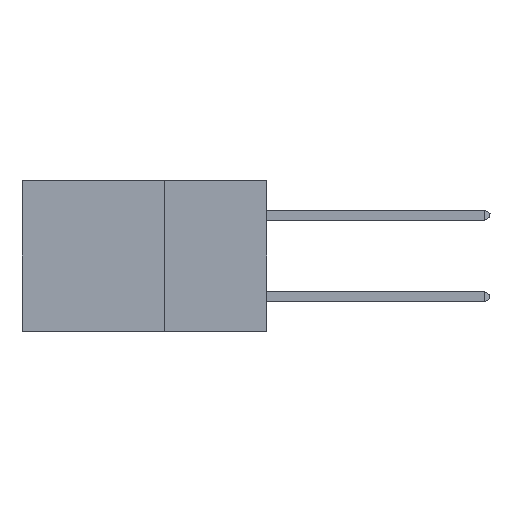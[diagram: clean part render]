
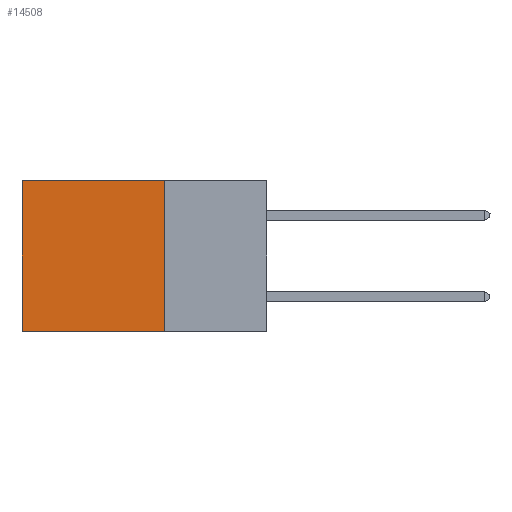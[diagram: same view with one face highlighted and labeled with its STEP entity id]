
A CAD part, left-side view. The second image highlights one B-rep face of the part: STEP entity #14508.
In plain terms, the highlighted planar face has unit normal (-1, 0, 0).
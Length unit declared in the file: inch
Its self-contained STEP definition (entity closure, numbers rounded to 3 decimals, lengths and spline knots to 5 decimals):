
#891 = LINE ( 'NONE', #15356, #12651 ) ;
#1156 = DIRECTION ( 'NONE',  ( 0., 1., 0. ) ) ;
#2074 = DIRECTION ( 'NONE',  ( 0., 1., 0. ) ) ;
#2158 = CARTESIAN_POINT ( 'NONE',  ( 0.2875, 0.25, 0. ) ) ;
#3663 = VECTOR ( 'NONE', #12455, 39.37008 ) ;
#4318 = CARTESIAN_POINT ( 'NONE',  ( 0.2875, 0.25, -0.37 ) ) ;
#5092 = LINE ( 'NONE', #8148, #12382 ) ;
#5104 = ORIENTED_EDGE ( 'NONE', *, *, #21086, .T. ) ;
#5555 = AXIS2_PLACEMENT_3D ( 'NONE', #7873, #11827, #15856 ) ;
#5577 = LINE ( 'NONE', #2158, #3663 ) ;
#7801 = VERTEX_POINT ( 'NONE', #24336 ) ;
#7873 = CARTESIAN_POINT ( 'NONE',  ( 0.2875, 0.25, 0. ) ) ;
#8148 = CARTESIAN_POINT ( 'NONE',  ( 0.2875, 0.25, 0. ) ) ;
#8924 = CARTESIAN_POINT ( 'NONE',  ( 0.2875, 0.25, -0.37 ) ) ;
#9270 = DIRECTION ( 'NONE',  ( 0., 0., -1. ) ) ;
#10845 = EDGE_CURVE ( 'NONE', #7801, #23779, #5092, .T. ) ;
#11282 = ORIENTED_EDGE ( 'NONE', *, *, #18665, .F. ) ;
#11827 = DIRECTION ( 'NONE',  ( 1., 0., 0. ) ) ;
#11918 = PLANE ( 'NONE',  #5555 ) ;
#12382 = VECTOR ( 'NONE', #2074, 39.37008 ) ;
#12455 = DIRECTION ( 'NONE',  ( 0., 0., -1. ) ) ;
#12651 = VECTOR ( 'NONE', #9270, 39.37008 ) ;
#12798 = FACE_OUTER_BOUND ( 'NONE', #18813, .T. ) ;
#14508 = ADVANCED_FACE ( 'NONE', ( #12798 ), #11918, .F. ) ;
#14721 = CARTESIAN_POINT ( 'NONE',  ( 0.2875, 0.6, 0. ) ) ;
#15114 = VECTOR ( 'NONE', #1156, 39.37008 ) ;
#15356 = CARTESIAN_POINT ( 'NONE',  ( 0.2875, 0.6, 0. ) ) ;
#15856 = DIRECTION ( 'NONE',  ( 0., 0., -1. ) ) ;
#16180 = ORIENTED_EDGE ( 'NONE', *, *, #24164, .F. ) ;
#18665 = EDGE_CURVE ( 'NONE', #19585, #23529, #24367, .T. ) ;
#18813 = EDGE_LOOP ( 'NONE', ( #5104, #11282, #16180, #20973 ) ) ;
#19585 = VERTEX_POINT ( 'NONE', #4318 ) ;
#20973 = ORIENTED_EDGE ( 'NONE', *, *, #10845, .T. ) ;
#21086 = EDGE_CURVE ( 'NONE', #23779, #23529, #891, .T. ) ;
#23529 = VERTEX_POINT ( 'NONE', #25286 ) ;
#23779 = VERTEX_POINT ( 'NONE', #14721 ) ;
#24164 = EDGE_CURVE ( 'NONE', #7801, #19585, #5577, .T. ) ;
#24336 = CARTESIAN_POINT ( 'NONE',  ( 0.2875, 0.25, 0. ) ) ;
#24367 = LINE ( 'NONE', #8924, #15114 ) ;
#25286 = CARTESIAN_POINT ( 'NONE',  ( 0.2875, 0.6, -0.37 ) ) ;
